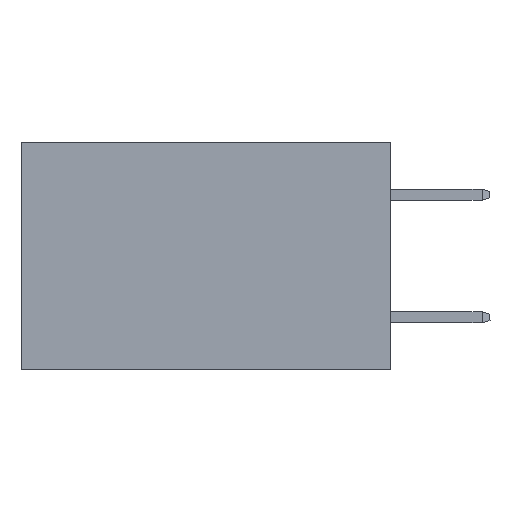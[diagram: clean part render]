
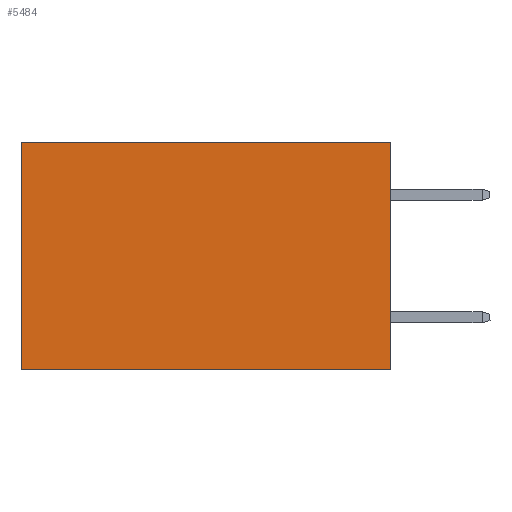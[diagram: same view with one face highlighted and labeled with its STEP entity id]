
A CAD part, left-side view. The second image highlights one B-rep face of the part: STEP entity #5484.
In plain terms, the highlighted planar face has unit normal (-1, 0, 0).
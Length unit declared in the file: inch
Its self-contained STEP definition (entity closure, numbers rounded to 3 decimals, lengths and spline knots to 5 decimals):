
#334 = LINE ( 'NONE', #3716, #4402 ) ;
#415 = VERTEX_POINT ( 'NONE', #2800 ) ;
#463 = VERTEX_POINT ( 'NONE', #6297 ) ;
#596 = EDGE_CURVE ( 'NONE', #415, #1949, #334, .T. ) ;
#720 = CARTESIAN_POINT ( 'NONE',  ( 0.2875, 0., 0. ) ) ;
#1007 = EDGE_CURVE ( 'NONE', #463, #3836, #7432, .T. ) ;
#1479 = ORIENTED_EDGE ( 'NONE', *, *, #4829, .F. ) ;
#1660 = ORIENTED_EDGE ( 'NONE', *, *, #1007, .T. ) ;
#1905 = CARTESIAN_POINT ( 'NONE',  ( 0.2875, 0., -0.37 ) ) ;
#1949 = VERTEX_POINT ( 'NONE', #1905 ) ;
#2312 = DIRECTION ( 'NONE',  ( 0., 0., -1. ) ) ;
#2410 = ORIENTED_EDGE ( 'NONE', *, *, #596, .F. ) ;
#2569 = EDGE_CURVE ( 'NONE', #415, #463, #7280, .T. ) ;
#2628 = CARTESIAN_POINT ( 'NONE',  ( 0.2875, 0.6, -0.37 ) ) ;
#2800 = CARTESIAN_POINT ( 'NONE',  ( 0.2875, 0., 0. ) ) ;
#2994 = PLANE ( 'NONE',  #6148 ) ;
#3516 = CARTESIAN_POINT ( 'NONE',  ( 0.2875, 0., 0. ) ) ;
#3524 = VECTOR ( 'NONE', #5667, 39.37008 ) ;
#3616 = VECTOR ( 'NONE', #7299, 39.37008 ) ;
#3716 = CARTESIAN_POINT ( 'NONE',  ( 0.2875, 0., 0. ) ) ;
#3836 = VERTEX_POINT ( 'NONE', #2628 ) ;
#3866 = LINE ( 'NONE', #6362, #3524 ) ;
#4402 = VECTOR ( 'NONE', #6569, 39.37008 ) ;
#4419 = DIRECTION ( 'NONE',  ( 1., 0., 0. ) ) ;
#4428 = EDGE_LOOP ( 'NONE', ( #1660, #1479, #2410, #7817 ) ) ;
#4601 = VECTOR ( 'NONE', #4871, 39.37008 ) ;
#4829 = EDGE_CURVE ( 'NONE', #1949, #3836, #3866, .T. ) ;
#4861 = FACE_OUTER_BOUND ( 'NONE', #4428, .T. ) ;
#4871 = DIRECTION ( 'NONE',  ( 0., 1., 0. ) ) ;
#5212 = CARTESIAN_POINT ( 'NONE',  ( 0.2875, 0.6, 0. ) ) ;
#5484 = ADVANCED_FACE ( 'NONE', ( #4861 ), #2994, .F. ) ;
#5667 = DIRECTION ( 'NONE',  ( 0., 1., 0. ) ) ;
#6148 = AXIS2_PLACEMENT_3D ( 'NONE', #720, #4419, #2312 ) ;
#6297 = CARTESIAN_POINT ( 'NONE',  ( 0.2875, 0.6, 0. ) ) ;
#6362 = CARTESIAN_POINT ( 'NONE',  ( 0.2875, 0., -0.37 ) ) ;
#6569 = DIRECTION ( 'NONE',  ( 0., 0., -1. ) ) ;
#7280 = LINE ( 'NONE', #3516, #4601 ) ;
#7299 = DIRECTION ( 'NONE',  ( 0., 0., -1. ) ) ;
#7432 = LINE ( 'NONE', #5212, #3616 ) ;
#7817 = ORIENTED_EDGE ( 'NONE', *, *, #2569, .T. ) ;
